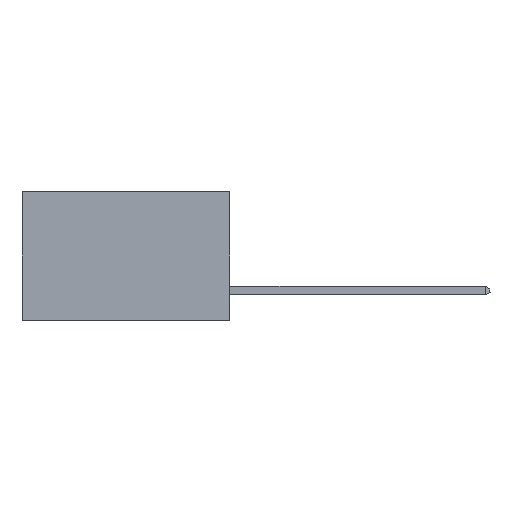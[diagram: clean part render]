
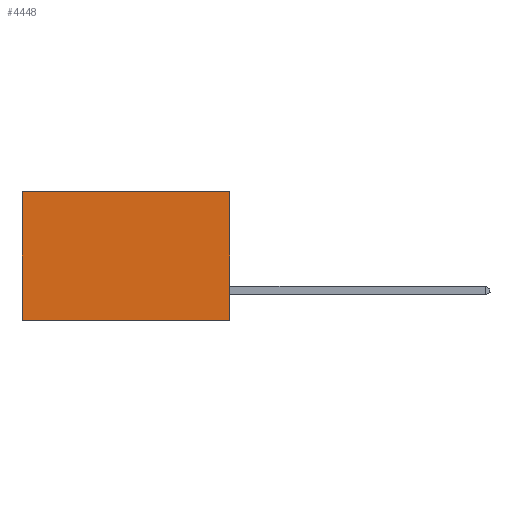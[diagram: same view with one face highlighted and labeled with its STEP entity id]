
A CAD part, left-side view. The second image highlights one B-rep face of the part: STEP entity #4448.
In plain terms, the highlighted planar face has unit normal (-1, 0, 0).
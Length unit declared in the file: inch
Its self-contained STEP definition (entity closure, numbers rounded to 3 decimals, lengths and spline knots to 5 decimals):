
#50 = DIRECTION ( 'NONE',  ( 0., 0., -1. ) ) ;
#1141 = VERTEX_POINT ( 'NONE', #12352 ) ;
#1213 = ORIENTED_EDGE ( 'NONE', *, *, #1311, .F. ) ;
#1311 = EDGE_CURVE ( 'NONE', #1141, #2006, #10418, .T. ) ;
#1423 = VECTOR ( 'NONE', #50, 39.37008 ) ;
#2006 = VERTEX_POINT ( 'NONE', #9011 ) ;
#3024 = CARTESIAN_POINT ( 'NONE',  ( 0.298, 0.6, 0. ) ) ;
#3376 = DIRECTION ( 'NONE',  ( 0., 1., 0. ) ) ;
#3691 = CARTESIAN_POINT ( 'NONE',  ( 0.298, 0., 0. ) ) ;
#3730 = VERTEX_POINT ( 'NONE', #3691 ) ;
#3873 = PLANE ( 'NONE',  #13148 ) ;
#4202 = ORIENTED_EDGE ( 'NONE', *, *, #14756, .T. ) ;
#4448 = ADVANCED_FACE ( 'NONE', ( #13007 ), #3873, .F. ) ;
#4814 = CARTESIAN_POINT ( 'NONE',  ( 0.298, 0.6, 0. ) ) ;
#5015 = VECTOR ( 'NONE', #3376, 39.37008 ) ;
#5347 = ORIENTED_EDGE ( 'NONE', *, *, #12587, .F. ) ;
#6564 = LINE ( 'NONE', #13279, #10496 ) ;
#8884 = CARTESIAN_POINT ( 'NONE',  ( 0.298, 0., 0. ) ) ;
#9011 = CARTESIAN_POINT ( 'NONE',  ( 0.298, 0.6, -0.37 ) ) ;
#9524 = CARTESIAN_POINT ( 'NONE',  ( 0.298, 0., -0.37 ) ) ;
#10418 = LINE ( 'NONE', #9524, #5015 ) ;
#10496 = VECTOR ( 'NONE', #13556, 39.37008 ) ;
#10968 = VERTEX_POINT ( 'NONE', #3024 ) ;
#12053 = DIRECTION ( 'NONE',  ( 0., 1., 0. ) ) ;
#12352 = CARTESIAN_POINT ( 'NONE',  ( 0.298, 0., -0.37 ) ) ;
#12587 = EDGE_CURVE ( 'NONE', #3730, #1141, #6564, .T. ) ;
#12680 = EDGE_CURVE ( 'NONE', #10968, #2006, #13431, .T. ) ;
#13007 = FACE_OUTER_BOUND ( 'NONE', #17900, .T. ) ;
#13116 = DIRECTION ( 'NONE',  ( 0., 0., -1. ) ) ;
#13148 = AXIS2_PLACEMENT_3D ( 'NONE', #16354, #17809, #13116 ) ;
#13279 = CARTESIAN_POINT ( 'NONE',  ( 0.298, 0., 0. ) ) ;
#13431 = LINE ( 'NONE', #4814, #1423 ) ;
#13556 = DIRECTION ( 'NONE',  ( 0., 0., -1. ) ) ;
#13937 = LINE ( 'NONE', #8884, #16624 ) ;
#14756 = EDGE_CURVE ( 'NONE', #3730, #10968, #13937, .T. ) ;
#16354 = CARTESIAN_POINT ( 'NONE',  ( 0.298, 0., 0. ) ) ;
#16624 = VECTOR ( 'NONE', #12053, 39.37008 ) ;
#17578 = ORIENTED_EDGE ( 'NONE', *, *, #12680, .T. ) ;
#17809 = DIRECTION ( 'NONE',  ( 1., 0., 0. ) ) ;
#17900 = EDGE_LOOP ( 'NONE', ( #17578, #1213, #5347, #4202 ) ) ;
